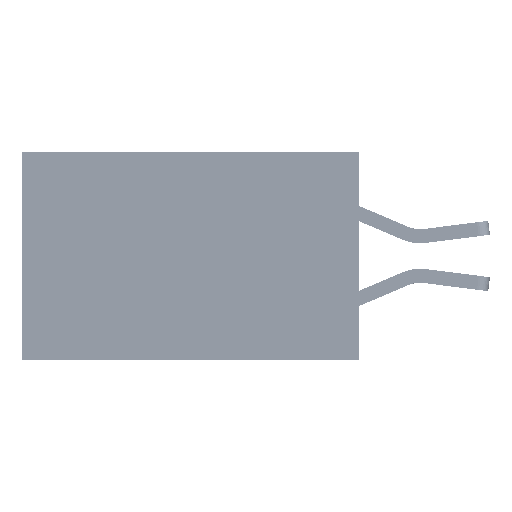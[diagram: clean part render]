
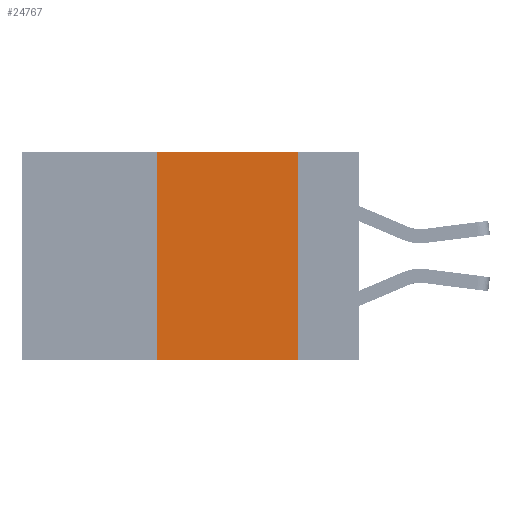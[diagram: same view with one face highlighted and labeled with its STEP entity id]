
A CAD part, left-side view. The second image highlights one B-rep face of the part: STEP entity #24767.
In plain terms, the highlighted planar face has unit normal (-1, 0, 0).
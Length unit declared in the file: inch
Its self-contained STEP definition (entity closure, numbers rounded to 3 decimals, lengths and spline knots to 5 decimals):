
#1048 = LINE ( 'NONE', #7646, #26707 ) ;
#1583 = LINE ( 'NONE', #39486, #31000 ) ;
#4019 = VERTEX_POINT ( 'NONE', #4236 ) ;
#4236 = CARTESIAN_POINT ( 'NONE',  ( 0., 0.11, -0.37 ) ) ;
#4468 = EDGE_LOOP ( 'NONE', ( #34178, #6822, #41854, #22164 ) ) ;
#6822 = ORIENTED_EDGE ( 'NONE', *, *, #21915, .F. ) ;
#7456 = LINE ( 'NONE', #37953, #48287 ) ;
#7646 = CARTESIAN_POINT ( 'NONE',  ( 0., 0.11, 0. ) ) ;
#7968 = VERTEX_POINT ( 'NONE', #8094 ) ;
#8094 = CARTESIAN_POINT ( 'NONE',  ( 0., 0.11, 0. ) ) ;
#9102 = EDGE_CURVE ( 'NONE', #30083, #30354, #27238, .T. ) ;
#10096 = AXIS2_PLACEMENT_3D ( 'NONE', #38154, #13504, #17822 ) ;
#10494 = DIRECTION ( 'NONE',  ( 0., 0., -1. ) ) ;
#13504 = DIRECTION ( 'NONE',  ( 1., 0., 0. ) ) ;
#16406 = VECTOR ( 'NONE', #22815, 39.37008 ) ;
#17822 = DIRECTION ( 'NONE',  ( 0., 0., -1. ) ) ;
#20041 = CARTESIAN_POINT ( 'NONE',  ( 0., 0.36, 0. ) ) ;
#21915 = EDGE_CURVE ( 'NONE', #30354, #7968, #1583, .T. ) ;
#21926 = CARTESIAN_POINT ( 'NONE',  ( 0., 0.36, 0. ) ) ;
#22164 = ORIENTED_EDGE ( 'NONE', *, *, #52334, .T. ) ;
#22197 = FACE_OUTER_BOUND ( 'NONE', #4468, .T. ) ;
#22815 = DIRECTION ( 'NONE',  ( 0., 0., 1. ) ) ;
#24767 = ADVANCED_FACE ( 'NONE', ( #22197 ), #45991, .F. ) ;
#26707 = VECTOR ( 'NONE', #10494, 39.37008 ) ;
#27238 = LINE ( 'NONE', #21926, #16406 ) ;
#27715 = DIRECTION ( 'NONE',  ( 0., -1., 0. ) ) ;
#30083 = VERTEX_POINT ( 'NONE', #42849 ) ;
#30354 = VERTEX_POINT ( 'NONE', #20041 ) ;
#31000 = VECTOR ( 'NONE', #27715, 39.37008 ) ;
#34178 = ORIENTED_EDGE ( 'NONE', *, *, #51689, .F. ) ;
#37953 = CARTESIAN_POINT ( 'NONE',  ( 0., 0.6, -0.37 ) ) ;
#38154 = CARTESIAN_POINT ( 'NONE',  ( 0., 0.6, 0. ) ) ;
#39486 = CARTESIAN_POINT ( 'NONE',  ( 0., 0.6, 0. ) ) ;
#41854 = ORIENTED_EDGE ( 'NONE', *, *, #9102, .F. ) ;
#42849 = CARTESIAN_POINT ( 'NONE',  ( 0., 0.36, -0.37 ) ) ;
#45962 = DIRECTION ( 'NONE',  ( 0., -1., 0. ) ) ;
#45991 = PLANE ( 'NONE',  #10096 ) ;
#48287 = VECTOR ( 'NONE', #45962, 39.37008 ) ;
#51689 = EDGE_CURVE ( 'NONE', #7968, #4019, #1048, .T. ) ;
#52334 = EDGE_CURVE ( 'NONE', #30083, #4019, #7456, .T. ) ;
